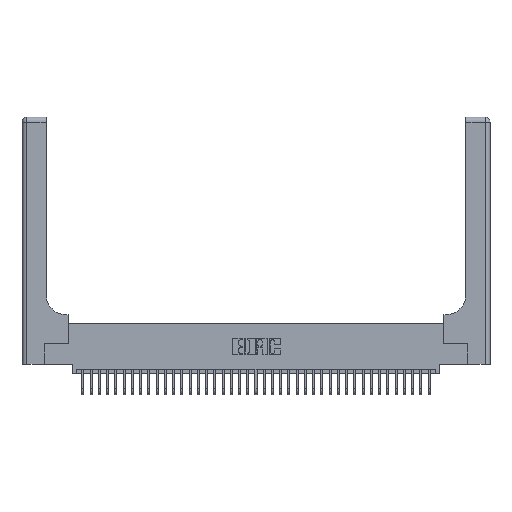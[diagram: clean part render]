
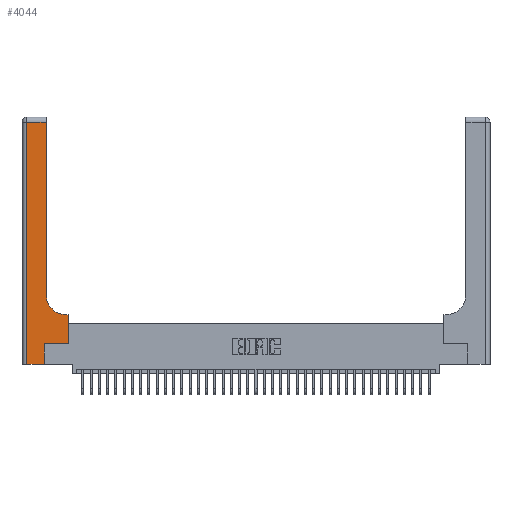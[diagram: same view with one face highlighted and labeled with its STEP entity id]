
A CAD part, top view. The second image highlights one B-rep face of the part: STEP entity #4044.
In plain terms, the highlighted planar face has unit normal (0, 0, 1).
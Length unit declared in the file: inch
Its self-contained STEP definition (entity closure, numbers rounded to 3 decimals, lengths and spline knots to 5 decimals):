
#496 = DIRECTION ( 'NONE',  ( -1., 0., 0. ) ) ;
#1069 = ORIENTED_EDGE ( 'NONE', *, *, #6884, .T. ) ;
#1223 = VERTEX_POINT ( 'NONE', #21169 ) ;
#1347 = EDGE_CURVE ( 'NONE', #34660, #19350, #14832, .T. ) ;
#3371 = ORIENTED_EDGE ( 'NONE', *, *, #11604, .T. ) ;
#3727 = FACE_OUTER_BOUND ( 'NONE', #20915, .T. ) ;
#3799 = VECTOR ( 'NONE', #31131, 39.37008 ) ;
#4044 = ADVANCED_FACE ( 'NONE', ( #3727 ), #22574, .F. ) ;
#4376 = LINE ( 'NONE', #16327, #5309 ) ;
#4758 = DIRECTION ( 'NONE',  ( 1., 0., 0. ) ) ;
#5258 = CARTESIAN_POINT ( 'NONE',  ( 0.06, 2.94, 0.37 ) ) ;
#5309 = VECTOR ( 'NONE', #30715, 39.37008 ) ;
#5413 = VECTOR ( 'NONE', #21320, 39.37008 ) ;
#5711 = CIRCLE ( 'NONE', #18022, 0.25 ) ;
#6884 = EDGE_CURVE ( 'NONE', #24838, #1223, #4376, .T. ) ;
#6943 = CARTESIAN_POINT ( 'NONE',  ( 0.5415, 0.85, 0.37 ) ) ;
#7150 = CARTESIAN_POINT ( 'NONE',  ( 0.269, 0.25, 0.37 ) ) ;
#8058 = CARTESIAN_POINT ( 'NONE',  ( 0., 3., 0.37 ) ) ;
#8173 = DIRECTION ( 'NONE',  ( 0., 1., 0. ) ) ;
#8882 = VERTEX_POINT ( 'NONE', #13275 ) ;
#9895 = DIRECTION ( 'NONE',  ( 1., 0., 0. ) ) ;
#9994 = DIRECTION ( 'NONE',  ( 1., 0., 0. ) ) ;
#10635 = LINE ( 'NONE', #10885, #3799 ) ;
#10885 = CARTESIAN_POINT ( 'NONE',  ( 0.269, 0., 0.37 ) ) ;
#11029 = DIRECTION ( 'NONE',  ( -1., 0., 0. ) ) ;
#11604 = EDGE_CURVE ( 'NONE', #32533, #21127, #5711, .T. ) ;
#11806 = CARTESIAN_POINT ( 'NONE',  ( 0.5585, 0.25, 0.37 ) ) ;
#13275 = CARTESIAN_POINT ( 'NONE',  ( 0.2915, 2.94, 0.37 ) ) ;
#13914 = CARTESIAN_POINT ( 'NONE',  ( 0.06, 3., 0.37 ) ) ;
#14117 = LINE ( 'NONE', #32863, #5413 ) ;
#14429 = CARTESIAN_POINT ( 'NONE',  ( 0.269, 0., 0.37 ) ) ;
#14832 = LINE ( 'NONE', #33224, #28362 ) ;
#15514 = LINE ( 'NONE', #22172, #24068 ) ;
#16327 = CARTESIAN_POINT ( 'NONE',  ( 0.5585, 0.25, 0.37 ) ) ;
#16660 = EDGE_CURVE ( 'NONE', #19350, #36845, #10635, .T. ) ;
#16740 = EDGE_CURVE ( 'NONE', #21127, #8882, #31004, .T. ) ;
#16818 = DIRECTION ( 'NONE',  ( 0., -1., 0. ) ) ;
#17014 = ORIENTED_EDGE ( 'NONE', *, *, #35063, .T. ) ;
#18022 = AXIS2_PLACEMENT_3D ( 'NONE', #6943, #27261, #9895 ) ;
#18753 = VERTEX_POINT ( 'NONE', #5258 ) ;
#19350 = VERTEX_POINT ( 'NONE', #14429 ) ;
#19586 = LINE ( 'NONE', #13914, #34100 ) ;
#20127 = ORIENTED_EDGE ( 'NONE', *, *, #16740, .T. ) ;
#20915 = EDGE_LOOP ( 'NONE', ( #20127, #37379, #21479, #23320, #37410, #17014, #1069, #26041, #3371 ) ) ;
#21127 = VERTEX_POINT ( 'NONE', #23730 ) ;
#21169 = CARTESIAN_POINT ( 'NONE',  ( 0.5585, 0.6, 0.37 ) ) ;
#21320 = DIRECTION ( 'NONE',  ( -1., 0., 0. ) ) ;
#21479 = ORIENTED_EDGE ( 'NONE', *, *, #22651, .T. ) ;
#21541 = AXIS2_PLACEMENT_3D ( 'NONE', #8058, #28372, #11029 ) ;
#22172 = CARTESIAN_POINT ( 'NONE',  ( 0.269, 0.25, 0.37 ) ) ;
#22574 = PLANE ( 'NONE',  #21541 ) ;
#22651 = EDGE_CURVE ( 'NONE', #18753, #34660, #19586, .T. ) ;
#23320 = ORIENTED_EDGE ( 'NONE', *, *, #1347, .T. ) ;
#23730 = CARTESIAN_POINT ( 'NONE',  ( 0.2915, 0.85, 0.37 ) ) ;
#24068 = VECTOR ( 'NONE', #4758, 39.37008 ) ;
#24229 = LINE ( 'NONE', #35282, #31014 ) ;
#24357 = EDGE_CURVE ( 'NONE', #8882, #18753, #14117, .T. ) ;
#24838 = VERTEX_POINT ( 'NONE', #11806 ) ;
#26041 = ORIENTED_EDGE ( 'NONE', *, *, #29171, .T. ) ;
#27261 = DIRECTION ( 'NONE',  ( 0., 0., -1. ) ) ;
#28362 = VECTOR ( 'NONE', #9994, 39.37008 ) ;
#28372 = DIRECTION ( 'NONE',  ( 0., 0., -1. ) ) ;
#29171 = EDGE_CURVE ( 'NONE', #1223, #32533, #24229, .T. ) ;
#30196 = CARTESIAN_POINT ( 'NONE',  ( 0.5415, 0.6, 0.37 ) ) ;
#30715 = DIRECTION ( 'NONE',  ( 0., 1., 0. ) ) ;
#31004 = LINE ( 'NONE', #37279, #31935 ) ;
#31014 = VECTOR ( 'NONE', #496, 39.37008 ) ;
#31131 = DIRECTION ( 'NONE',  ( 0., 1., 0. ) ) ;
#31198 = CARTESIAN_POINT ( 'NONE',  ( 0.06, 0., 0.37 ) ) ;
#31935 = VECTOR ( 'NONE', #8173, 39.37008 ) ;
#32533 = VERTEX_POINT ( 'NONE', #30196 ) ;
#32863 = CARTESIAN_POINT ( 'NONE',  ( 0., 2.94, 0.37 ) ) ;
#33224 = CARTESIAN_POINT ( 'NONE',  ( 0., 0., 0.37 ) ) ;
#34100 = VECTOR ( 'NONE', #16818, 39.37008 ) ;
#34660 = VERTEX_POINT ( 'NONE', #31198 ) ;
#35063 = EDGE_CURVE ( 'NONE', #36845, #24838, #15514, .T. ) ;
#35282 = CARTESIAN_POINT ( 'NONE',  ( 0.2915, 0.6, 0.37 ) ) ;
#36845 = VERTEX_POINT ( 'NONE', #7150 ) ;
#37279 = CARTESIAN_POINT ( 'NONE',  ( 0.2915, 3., 0.37 ) ) ;
#37379 = ORIENTED_EDGE ( 'NONE', *, *, #24357, .T. ) ;
#37410 = ORIENTED_EDGE ( 'NONE', *, *, #16660, .T. ) ;
